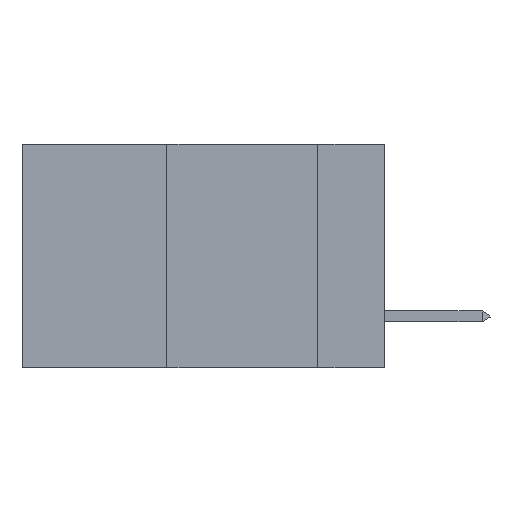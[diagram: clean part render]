
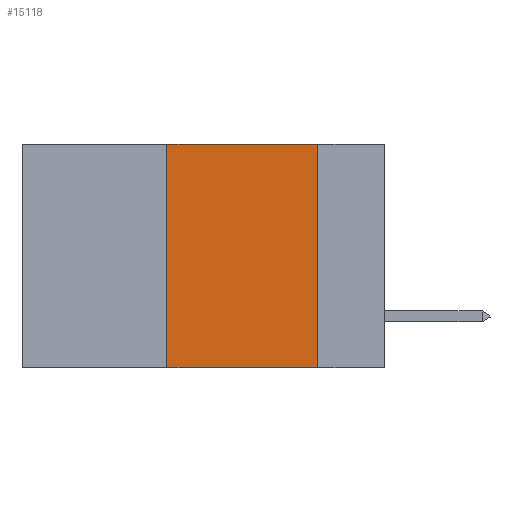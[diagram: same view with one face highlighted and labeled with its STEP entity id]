
A CAD part, left-side view. The second image highlights one B-rep face of the part: STEP entity #15118.
In plain terms, the highlighted planar face has unit normal (-1, 0, 0).
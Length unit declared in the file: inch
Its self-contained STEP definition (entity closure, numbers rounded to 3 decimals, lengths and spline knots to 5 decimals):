
#876 = FACE_OUTER_BOUND ( 'NONE', #5848, .T. ) ;
#1645 = ORIENTED_EDGE ( 'NONE', *, *, #20961, .T. ) ;
#1877 = CARTESIAN_POINT ( 'NONE',  ( 0., 0.36, 0. ) ) ;
#2048 = DIRECTION ( 'NONE',  ( 1., 0., 0. ) ) ;
#3465 = VERTEX_POINT ( 'NONE', #10264 ) ;
#5468 = VECTOR ( 'NONE', #13289, 39.37008 ) ;
#5601 = CARTESIAN_POINT ( 'NONE',  ( 0., 0.11, 0. ) ) ;
#5848 = EDGE_LOOP ( 'NONE', ( #8349, #13742, #14665, #1645 ) ) ;
#6353 = VECTOR ( 'NONE', #6633, 39.37008 ) ;
#6633 = DIRECTION ( 'NONE',  ( 0., -1., 0. ) ) ;
#7407 = EDGE_CURVE ( 'NONE', #16107, #14815, #7869, .T. ) ;
#7869 = LINE ( 'NONE', #5601, #12100 ) ;
#8349 = ORIENTED_EDGE ( 'NONE', *, *, #7407, .F. ) ;
#9490 = CARTESIAN_POINT ( 'NONE',  ( 0., 0.11, 0. ) ) ;
#9602 = CARTESIAN_POINT ( 'NONE',  ( 0., 0.6, -0.37 ) ) ;
#9960 = VERTEX_POINT ( 'NONE', #1877 ) ;
#10264 = CARTESIAN_POINT ( 'NONE',  ( 0., 0.36, -0.37 ) ) ;
#10275 = VECTOR ( 'NONE', #19758, 39.37008 ) ;
#10843 = LINE ( 'NONE', #12703, #10275 ) ;
#10887 = LINE ( 'NONE', #9602, #5468 ) ;
#12100 = VECTOR ( 'NONE', #23230, 39.37008 ) ;
#12703 = CARTESIAN_POINT ( 'NONE',  ( 0., 0.36, 0. ) ) ;
#12978 = CARTESIAN_POINT ( 'NONE',  ( 0., 0.6, 0. ) ) ;
#13289 = DIRECTION ( 'NONE',  ( 0., -1., 0. ) ) ;
#13742 = ORIENTED_EDGE ( 'NONE', *, *, #16363, .F. ) ;
#14665 = ORIENTED_EDGE ( 'NONE', *, *, #17887, .F. ) ;
#14768 = DIRECTION ( 'NONE',  ( 0., 0., -1. ) ) ;
#14815 = VERTEX_POINT ( 'NONE', #22567 ) ;
#15118 = ADVANCED_FACE ( 'NONE', ( #876 ), #21633, .F. ) ;
#15257 = AXIS2_PLACEMENT_3D ( 'NONE', #12978, #2048, #14768 ) ;
#16107 = VERTEX_POINT ( 'NONE', #9490 ) ;
#16363 = EDGE_CURVE ( 'NONE', #9960, #16107, #20497, .T. ) ;
#17887 = EDGE_CURVE ( 'NONE', #3465, #9960, #10843, .T. ) ;
#19758 = DIRECTION ( 'NONE',  ( 0., 0., 1. ) ) ;
#20497 = LINE ( 'NONE', #20704, #6353 ) ;
#20704 = CARTESIAN_POINT ( 'NONE',  ( 0., 0.6, 0. ) ) ;
#20961 = EDGE_CURVE ( 'NONE', #3465, #14815, #10887, .T. ) ;
#21633 = PLANE ( 'NONE',  #15257 ) ;
#22567 = CARTESIAN_POINT ( 'NONE',  ( 0., 0.11, -0.37 ) ) ;
#23230 = DIRECTION ( 'NONE',  ( 0., 0., -1. ) ) ;
